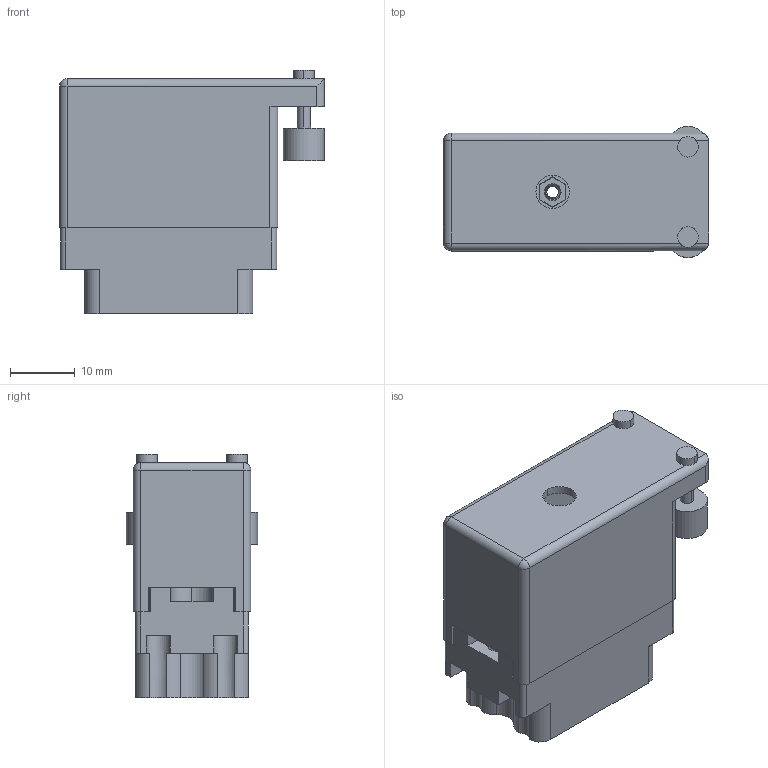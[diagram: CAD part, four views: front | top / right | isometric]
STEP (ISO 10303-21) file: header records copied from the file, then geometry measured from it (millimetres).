
FILE_DESCRIPTION (( 'STEP AP203' ), '1' );
FILE_NAME ('519-014-500-326.STEP', '2020-03-02T20:12:41', ( '' ), ( '' ), 'SwSTEP 2.0', 'SolidWorks 2016', '' );
FILE_SCHEMA (( 'CONFIG_CONTROL_DESIGN' ));
Length unit declared in the file: inch
Products named in the file (5): 516-230-001_Plastic - 020 Side Entry; 519 Plug Insulator_014; 519-014-500-326; 516-252-025-100_516-252-025-100; 516-292-001_500 Contact
Assembly tree (17 placements, depth 2):
  519-014-500-326
    519 Plug Insulator_014
    516-292-001_500 Contact  x14
    516-252-025-100_516-252-025-100
    516-230-001_Plastic - 020 Side Entry
Bounding box: 40.87 x 20.24 x 37.52 mm (x, y, z)
Volume: 9424.2 mm3; surface area: 15044.2 mm2
Topology: 17 solids, 17 shells, 1676 faces, 4846 edges, 3211 vertices
Faces by surface type: plane 971, cylinder 605, bspline 87, cone 11, sphere 2
Entity records: 26406 total; most frequent: CARTESIAN_POINT 7032, ORIENTED_EDGE 3968, DIRECTION 3821, EDGE_CURVE 1984, LINE 1353, VECTOR 1353, VERTEX_POINT 1313, AXIS2_PLACEMENT_3D 1234
